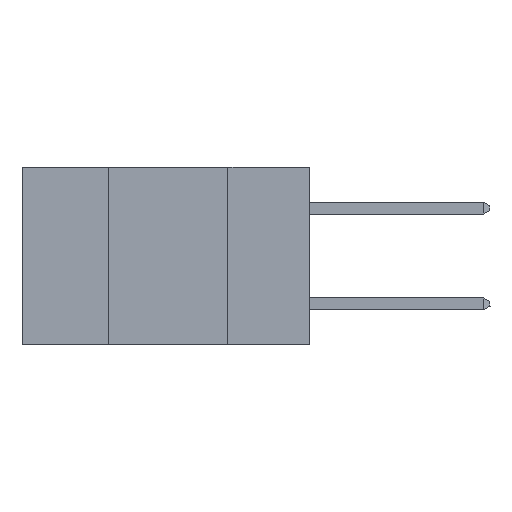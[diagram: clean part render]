
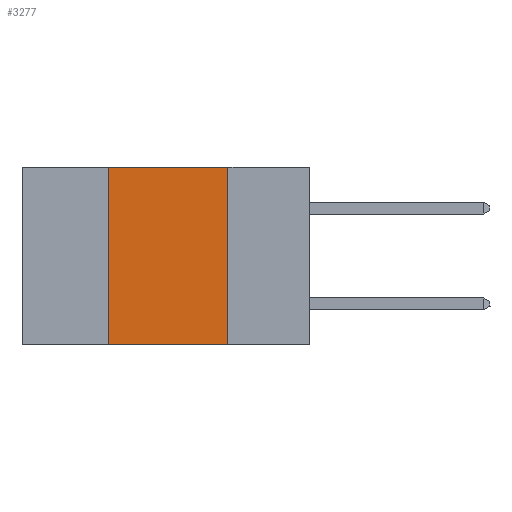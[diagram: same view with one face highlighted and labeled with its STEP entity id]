
A CAD part, left-side view. The second image highlights one B-rep face of the part: STEP entity #3277.
In plain terms, the highlighted planar face has unit normal (-1, 0, 0).
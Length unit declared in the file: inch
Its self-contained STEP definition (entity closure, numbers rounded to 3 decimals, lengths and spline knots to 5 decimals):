
#312 = VECTOR ( 'NONE', #7786, 39.37008 ) ;
#1035 = CARTESIAN_POINT ( 'NONE',  ( 0., 0.42, -0.37 ) ) ;
#1404 = CARTESIAN_POINT ( 'NONE',  ( 0., 0.6, 0. ) ) ;
#1681 = CARTESIAN_POINT ( 'NONE',  ( 0., 0.42, 0. ) ) ;
#2366 = VERTEX_POINT ( 'NONE', #20042 ) ;
#3136 = AXIS2_PLACEMENT_3D ( 'NONE', #1404, #3372, #21543 ) ;
#3271 = EDGE_CURVE ( 'NONE', #8244, #2366, #5723, .T. ) ;
#3277 = ADVANCED_FACE ( 'NONE', ( #6011 ), #16042, .F. ) ;
#3372 = DIRECTION ( 'NONE',  ( 1., 0., 0. ) ) ;
#4628 = DIRECTION ( 'NONE',  ( 0., -1., 0. ) ) ;
#5723 = LINE ( 'NONE', #23551, #10374 ) ;
#5990 = EDGE_CURVE ( 'NONE', #11234, #2366, #6223, .T. ) ;
#6011 = FACE_OUTER_BOUND ( 'NONE', #19303, .T. ) ;
#6223 = LINE ( 'NONE', #21383, #20413 ) ;
#6978 = CARTESIAN_POINT ( 'NONE',  ( 0., 0.6, 0. ) ) ;
#7786 = DIRECTION ( 'NONE',  ( 0., 0., 1. ) ) ;
#8244 = VERTEX_POINT ( 'NONE', #10916 ) ;
#8615 = DIRECTION ( 'NONE',  ( 0., 0., -1. ) ) ;
#10374 = VECTOR ( 'NONE', #8615, 39.37008 ) ;
#10804 = ORIENTED_EDGE ( 'NONE', *, *, #14500, .F. ) ;
#10916 = CARTESIAN_POINT ( 'NONE',  ( 0., 0.17, 0. ) ) ;
#11234 = VERTEX_POINT ( 'NONE', #1035 ) ;
#11582 = CARTESIAN_POINT ( 'NONE',  ( 0., 0.42, 0. ) ) ;
#11865 = ORIENTED_EDGE ( 'NONE', *, *, #3271, .F. ) ;
#12399 = DIRECTION ( 'NONE',  ( 0., -1., 0. ) ) ;
#14497 = LINE ( 'NONE', #6978, #23755 ) ;
#14500 = EDGE_CURVE ( 'NONE', #15297, #8244, #14497, .T. ) ;
#15297 = VERTEX_POINT ( 'NONE', #1681 ) ;
#16042 = PLANE ( 'NONE',  #3136 ) ;
#16312 = LINE ( 'NONE', #11582, #312 ) ;
#18646 = ORIENTED_EDGE ( 'NONE', *, *, #20996, .F. ) ;
#19303 = EDGE_LOOP ( 'NONE', ( #11865, #10804, #18646, #21545 ) ) ;
#20042 = CARTESIAN_POINT ( 'NONE',  ( 0., 0.17, -0.37 ) ) ;
#20413 = VECTOR ( 'NONE', #4628, 39.37008 ) ;
#20996 = EDGE_CURVE ( 'NONE', #11234, #15297, #16312, .T. ) ;
#21383 = CARTESIAN_POINT ( 'NONE',  ( 0., 0.6, -0.37 ) ) ;
#21543 = DIRECTION ( 'NONE',  ( 0., 0., -1. ) ) ;
#21545 = ORIENTED_EDGE ( 'NONE', *, *, #5990, .T. ) ;
#23551 = CARTESIAN_POINT ( 'NONE',  ( 0., 0.17, 0. ) ) ;
#23755 = VECTOR ( 'NONE', #12399, 39.37008 ) ;
